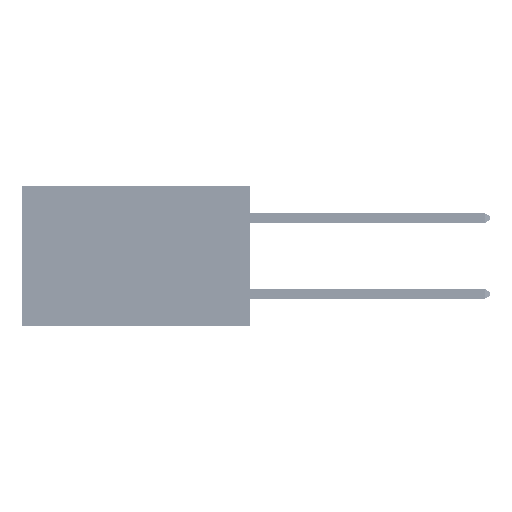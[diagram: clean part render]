
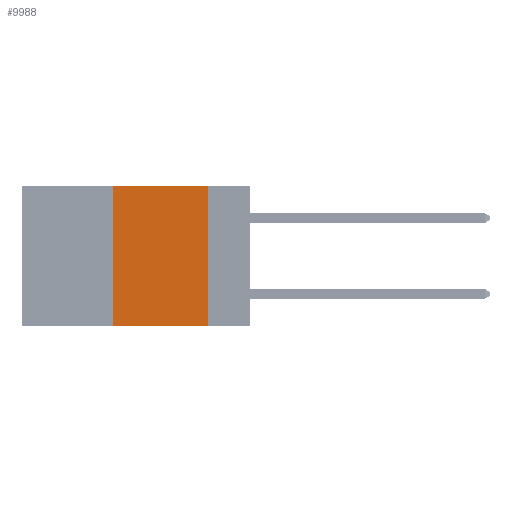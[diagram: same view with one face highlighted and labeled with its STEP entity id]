
A CAD part, left-side view. The second image highlights one B-rep face of the part: STEP entity #9988.
In plain terms, the highlighted planar face has unit normal (-1, 0, 0).
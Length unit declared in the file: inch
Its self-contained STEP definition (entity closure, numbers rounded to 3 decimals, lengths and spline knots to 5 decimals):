
#2822 = DIRECTION ( 'NONE',  ( 0., 0., -1. ) ) ;
#3679 = LINE ( 'NONE', #22236, #44782 ) ;
#4329 = LINE ( 'NONE', #40921, #16467 ) ;
#7342 = ORIENTED_EDGE ( 'NONE', *, *, #27165, .F. ) ;
#9917 = FACE_OUTER_BOUND ( 'NONE', #49976, .T. ) ;
#9988 = ADVANCED_FACE ( 'NONE', ( #9917 ), #14889, .F. ) ;
#10792 = EDGE_CURVE ( 'NONE', #23501, #37726, #4329, .T. ) ;
#11019 = CARTESIAN_POINT ( 'NONE',  ( 0., 0.6, 0. ) ) ;
#11137 = AXIS2_PLACEMENT_3D ( 'NONE', #11019, #18626, #26908 ) ;
#14113 = VECTOR ( 'NONE', #28571, 39.37008 ) ;
#14889 = PLANE ( 'NONE',  #11137 ) ;
#16467 = VECTOR ( 'NONE', #35845, 39.37008 ) ;
#18084 = EDGE_CURVE ( 'NONE', #23501, #19669, #47949, .T. ) ;
#18626 = DIRECTION ( 'NONE',  ( 1., 0., 0. ) ) ;
#19669 = VERTEX_POINT ( 'NONE', #21814 ) ;
#20949 = DIRECTION ( 'NONE',  ( 0., -1., 0. ) ) ;
#21814 = CARTESIAN_POINT ( 'NONE',  ( 0., 0.11, -0.37 ) ) ;
#22236 = CARTESIAN_POINT ( 'NONE',  ( 0., 0.11, 0. ) ) ;
#22275 = CARTESIAN_POINT ( 'NONE',  ( 0., 0.36, -0.37 ) ) ;
#23501 = VERTEX_POINT ( 'NONE', #22275 ) ;
#25722 = ORIENTED_EDGE ( 'NONE', *, *, #26761, .F. ) ;
#26761 = EDGE_CURVE ( 'NONE', #28957, #19669, #3679, .T. ) ;
#26908 = DIRECTION ( 'NONE',  ( 0., 0., -1. ) ) ;
#27165 = EDGE_CURVE ( 'NONE', #37726, #28957, #37480, .T. ) ;
#27941 = CARTESIAN_POINT ( 'NONE',  ( 0., 0.11, 0. ) ) ;
#28571 = DIRECTION ( 'NONE',  ( 0., -1., 0. ) ) ;
#28957 = VERTEX_POINT ( 'NONE', #27941 ) ;
#34162 = ORIENTED_EDGE ( 'NONE', *, *, #10792, .F. ) ;
#35845 = DIRECTION ( 'NONE',  ( 0., 0., 1. ) ) ;
#36673 = CARTESIAN_POINT ( 'NONE',  ( 0., 0.6, 0. ) ) ;
#37363 = CARTESIAN_POINT ( 'NONE',  ( 0., 0.36, 0. ) ) ;
#37480 = LINE ( 'NONE', #36673, #38052 ) ;
#37726 = VERTEX_POINT ( 'NONE', #37363 ) ;
#38052 = VECTOR ( 'NONE', #20949, 39.37008 ) ;
#40921 = CARTESIAN_POINT ( 'NONE',  ( 0., 0.36, 0. ) ) ;
#44782 = VECTOR ( 'NONE', #2822, 39.37008 ) ;
#47949 = LINE ( 'NONE', #48131, #14113 ) ;
#48131 = CARTESIAN_POINT ( 'NONE',  ( 0., 0.6, -0.37 ) ) ;
#49006 = ORIENTED_EDGE ( 'NONE', *, *, #18084, .T. ) ;
#49976 = EDGE_LOOP ( 'NONE', ( #25722, #7342, #34162, #49006 ) ) ;
